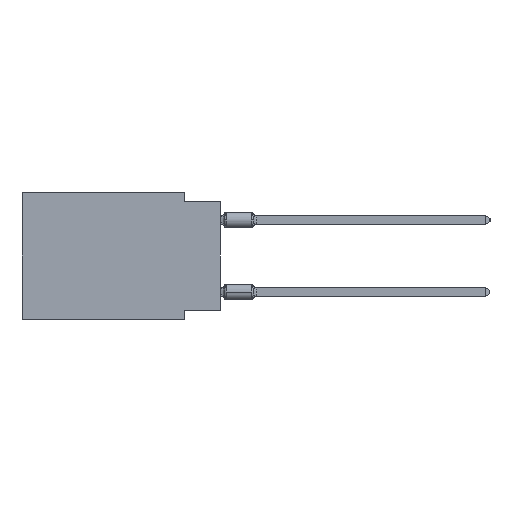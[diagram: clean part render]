
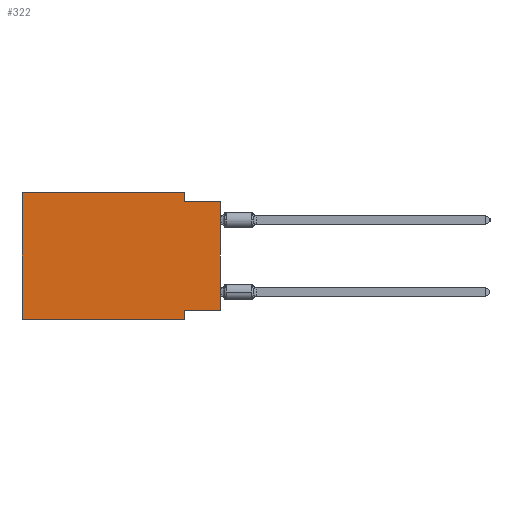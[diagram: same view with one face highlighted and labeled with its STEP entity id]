
A CAD part, left-side view. The second image highlights one B-rep face of the part: STEP entity #322.
In plain terms, the highlighted planar face has unit normal (-1, 0, 0).
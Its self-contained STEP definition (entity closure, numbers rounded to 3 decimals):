
#184 = VECTOR ( 'NONE', #23874, 1000. ) ;
#258 = CARTESIAN_POINT ( 'NONE',  ( 0., 0., -8.255 ) ) ;
#277 = EDGE_CURVE ( 'NONE', #433, #24013, #4786, .T. ) ;
#322 = ADVANCED_FACE ( 'NONE', ( #18559 ), #13886, .F. ) ;
#433 = VERTEX_POINT ( 'NONE', #12606 ) ;
#1560 = DIRECTION ( 'NONE',  ( 0., -1., 0. ) ) ;
#2267 = LINE ( 'NONE', #17127, #3106 ) ;
#2587 = CARTESIAN_POINT ( 'NONE',  ( 0., 2.54, -0.635 ) ) ;
#3106 = VECTOR ( 'NONE', #14481, 1000. ) ;
#4123 = CARTESIAN_POINT ( 'NONE',  ( 0., 2.54, -8.89 ) ) ;
#4786 = LINE ( 'NONE', #23725, #184 ) ;
#4908 = VERTEX_POINT ( 'NONE', #10066 ) ;
#5583 = ORIENTED_EDGE ( 'NONE', *, *, #14163, .T. ) ;
#6832 = CARTESIAN_POINT ( 'NONE',  ( 0., 2.54, -8.255 ) ) ;
#6911 = ORIENTED_EDGE ( 'NONE', *, *, #21035, .F. ) ;
#6966 = CARTESIAN_POINT ( 'NONE',  ( 0., 2.54, -8.89 ) ) ;
#8068 = VECTOR ( 'NONE', #24194, 1000. ) ;
#10066 = CARTESIAN_POINT ( 'NONE',  ( 0., 13.97, 0. ) ) ;
#10208 = ORIENTED_EDGE ( 'NONE', *, *, #22779, .F. ) ;
#10651 = VERTEX_POINT ( 'NONE', #15242 ) ;
#11112 = LINE ( 'NONE', #15807, #22593 ) ;
#11529 = EDGE_LOOP ( 'NONE', ( #16258, #22446, #20285, #17693, #10208, #5583, #20101, #6911 ) ) ;
#11538 = VECTOR ( 'NONE', #16668, 1000. ) ;
#11625 = CARTESIAN_POINT ( 'NONE',  ( 0., 13.97, -8.89 ) ) ;
#12606 = CARTESIAN_POINT ( 'NONE',  ( 0., 0., -8.255 ) ) ;
#13886 = PLANE ( 'NONE',  #23193 ) ;
#14163 = EDGE_CURVE ( 'NONE', #21903, #24460, #18806, .T. ) ;
#14481 = DIRECTION ( 'NONE',  ( 0., 0., 1. ) ) ;
#14621 = VECTOR ( 'NONE', #28284, 1000. ) ;
#15035 = VERTEX_POINT ( 'NONE', #6832 ) ;
#15242 = CARTESIAN_POINT ( 'NONE',  ( 0., 2.54, 0. ) ) ;
#15807 = CARTESIAN_POINT ( 'NONE',  ( 0., 13.97, 0. ) ) ;
#16258 = ORIENTED_EDGE ( 'NONE', *, *, #277, .T. ) ;
#16668 = DIRECTION ( 'NONE',  ( 0., 0., -1. ) ) ;
#17127 = CARTESIAN_POINT ( 'NONE',  ( 0., 13.97, 0. ) ) ;
#17133 = CARTESIAN_POINT ( 'NONE',  ( 0., 0., -0.635 ) ) ;
#17611 = VERTEX_POINT ( 'NONE', #2587 ) ;
#17693 = ORIENTED_EDGE ( 'NONE', *, *, #20306, .F. ) ;
#18559 = FACE_OUTER_BOUND ( 'NONE', #11529, .T. ) ;
#18806 = LINE ( 'NONE', #11625, #26845 ) ;
#20101 = ORIENTED_EDGE ( 'NONE', *, *, #21524, .F. ) ;
#20204 = EDGE_CURVE ( 'NONE', #10651, #17611, #21401, .T. ) ;
#20285 = ORIENTED_EDGE ( 'NONE', *, *, #20204, .F. ) ;
#20306 = EDGE_CURVE ( 'NONE', #4908, #10651, #11112, .T. ) ;
#21035 = EDGE_CURVE ( 'NONE', #433, #15035, #21698, .T. ) ;
#21401 = LINE ( 'NONE', #28606, #14621 ) ;
#21524 = EDGE_CURVE ( 'NONE', #15035, #24460, #30766, .T. ) ;
#21698 = LINE ( 'NONE', #258, #8068 ) ;
#21903 = VERTEX_POINT ( 'NONE', #26161 ) ;
#22446 = ORIENTED_EDGE ( 'NONE', *, *, #23745, .F. ) ;
#22593 = VECTOR ( 'NONE', #1560, 1000. ) ;
#22779 = EDGE_CURVE ( 'NONE', #21903, #4908, #2267, .T. ) ;
#23193 = AXIS2_PLACEMENT_3D ( 'NONE', #25605, #30632, #23412 ) ;
#23412 = DIRECTION ( 'NONE',  ( 0., 0., -1. ) ) ;
#23725 = CARTESIAN_POINT ( 'NONE',  ( 0., 0., 0. ) ) ;
#23745 = EDGE_CURVE ( 'NONE', #17611, #24013, #30191, .T. ) ;
#23874 = DIRECTION ( 'NONE',  ( 0., 0., 1. ) ) ;
#24013 = VERTEX_POINT ( 'NONE', #17133 ) ;
#24194 = DIRECTION ( 'NONE',  ( 0., 1., 0. ) ) ;
#24460 = VERTEX_POINT ( 'NONE', #4123 ) ;
#24925 = VECTOR ( 'NONE', #28413, 1000. ) ;
#25605 = CARTESIAN_POINT ( 'NONE',  ( 0., 13.97, 0. ) ) ;
#26161 = CARTESIAN_POINT ( 'NONE',  ( 0., 13.97, -8.89 ) ) ;
#26845 = VECTOR ( 'NONE', #30251, 1000. ) ;
#28284 = DIRECTION ( 'NONE',  ( 0., 0., -1. ) ) ;
#28413 = DIRECTION ( 'NONE',  ( 0., -1., 0. ) ) ;
#28606 = CARTESIAN_POINT ( 'NONE',  ( 0., 2.54, 0. ) ) ;
#29724 = CARTESIAN_POINT ( 'NONE',  ( 0., 0., -0.635 ) ) ;
#30191 = LINE ( 'NONE', #29724, #24925 ) ;
#30251 = DIRECTION ( 'NONE',  ( 0., -1., 0. ) ) ;
#30632 = DIRECTION ( 'NONE',  ( 1., 0., 0. ) ) ;
#30766 = LINE ( 'NONE', #6966, #11538 ) ;
